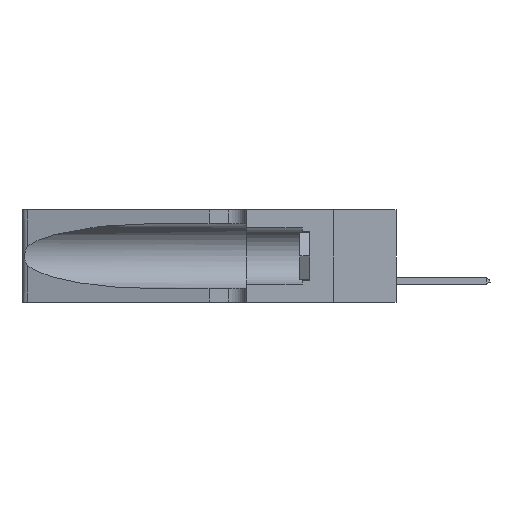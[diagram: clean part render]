
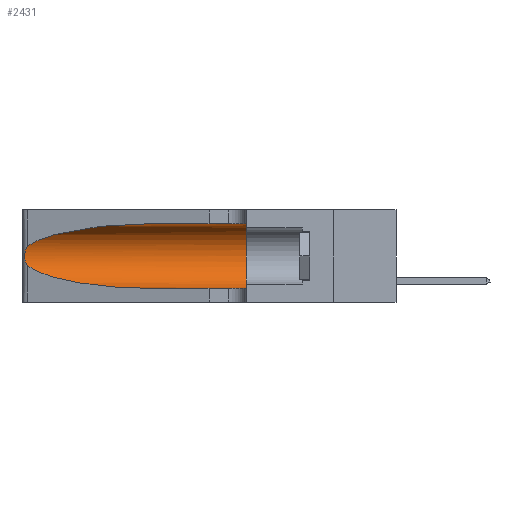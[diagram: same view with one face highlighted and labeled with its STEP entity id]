
A CAD part, left-side view. The second image highlights one B-rep face of the part: STEP entity #2431.
In plain terms, the highlighted cylindrical face has radius 3.308 mm (diameter 6.617 mm), a partial arc.
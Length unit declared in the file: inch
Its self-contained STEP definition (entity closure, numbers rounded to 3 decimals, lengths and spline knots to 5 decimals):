
#543 = CARTESIAN_POINT ( 'NONE',  ( 0.25856, 1.23593, 0.16098 ) ) ;
#841 = CARTESIAN_POINT ( 'NONE',  ( 0.25555, 1.22994, 0.2215 ) ) ;
#2431 = ADVANCED_FACE ( 'NONE', ( #20573 ), #27741, .F. ) ;
#2464 = EDGE_CURVE ( 'NONE', #37446, #22092, #39561, .T. ) ;
#2761 = EDGE_CURVE ( 'NONE', #19923, #37446, #9212, .T. ) ;
#3062 = CARTESIAN_POINT ( 'NONE',  ( 0.1305, 0.35, 0.185 ) ) ;
#3787 = CARTESIAN_POINT ( 'NONE',  ( 0.25639, 1.23184, 0.21858 ) ) ;
#3931 = CARTESIAN_POINT ( 'NONE',  ( 0.25639, 1.23186, 0.15144 ) ) ;
#4174 = VERTEX_POINT ( 'NONE', #24287 ) ;
#5239 = EDGE_CURVE ( 'NONE', #22092, #4174, #22584, .T. ) ;
#5716 = VECTOR ( 'NONE', #24794, 39.37008 ) ;
#5760 = VECTOR ( 'NONE', #39925, 39.37008 ) ;
#7243 = CARTESIAN_POINT ( 'NONE',  ( 0.26075, 1.23896, 0.178 ) ) ;
#7381 = CARTESIAN_POINT ( 'NONE',  ( 0.26017, 1.23833, 0.17102 ) ) ;
#7529 = CARTESIAN_POINT ( 'NONE',  ( 0.25487, 1.22718, 0.14631 ) ) ;
#9212 =( BOUNDED_CURVE ( )  B_SPLINE_CURVE ( 3, ( #34380, #21546, #33027, #35935 ),
 .UNSPECIFIED., .F., .F. ) 
 B_SPLINE_CURVE_WITH_KNOTS ( ( 4, 4 ),
 ( 1.5708, 2.84003 ),
 .UNSPECIFIED. ) 
 CURVE ( )  GEOMETRIC_REPRESENTATION_ITEM ( )  RATIONAL_B_SPLINE_CURVE ( ( 1., 0.87, 0.87, 1. ) ) 
 REPRESENTATION_ITEM ( '' )  );
#10047 = ORIENTED_EDGE ( 'NONE', *, *, #25328, .T. ) ;
#10255 = DIRECTION ( 'NONE',  ( 0., 0., -1. ) ) ;
#10950 = CARTESIAN_POINT ( 'NONE',  ( 0.26075, 1.23896, 0.19203 ) ) ;
#12093 = CARTESIAN_POINT ( 'NONE',  ( 0.25487, 1.22718, 0.14631 ) ) ;
#12885 = CARTESIAN_POINT ( 'NONE',  ( 0.18966, 0.96281, 0.05475 ) ) ;
#13194 = DIRECTION ( 'NONE',  ( 0., 1., 0. ) ) ;
#13235 = CARTESIAN_POINT ( 'NONE',  ( 0.1305, 0.72297, 0.05475 ) ) ;
#13467 = ORIENTED_EDGE ( 'NONE', *, *, #19697, .F. ) ;
#14350 = CARTESIAN_POINT ( 'NONE',  ( 0.1305, 1.61858, 0.31525 ) ) ;
#16114 = ORIENTED_EDGE ( 'NONE', *, *, #2761, .T. ) ;
#17792 = CARTESIAN_POINT ( 'NONE',  ( 0.1305, 0.35, 0.31525 ) ) ;
#19623 = CIRCLE ( 'NONE', #22662, 0.13025 ) ;
#19697 = EDGE_CURVE ( 'NONE', #19923, #32440, #25213, .T. ) ;
#19923 = VERTEX_POINT ( 'NONE', #24162 ) ;
#20248 = CARTESIAN_POINT ( 'NONE',  ( 0.25787, 1.23484, 0.2124 ) ) ;
#20573 = FACE_OUTER_BOUND ( 'NONE', #28814, .T. ) ;
#21546 = CARTESIAN_POINT ( 'NONE',  ( 0.18966, 0.96281, 0.31525 ) ) ;
#21591 = ORIENTED_EDGE ( 'NONE', *, *, #2464, .T. ) ;
#22092 = VERTEX_POINT ( 'NONE', #38915 ) ;
#22584 =( BOUNDED_CURVE ( )  B_SPLINE_CURVE ( 3, ( #12093, #30904, #12885, #13235 ),
 .UNSPECIFIED., .F., .F. ) 
 B_SPLINE_CURVE_WITH_KNOTS ( ( 4, 4 ),
 ( 3.44316, 4.71239 ),
 .UNSPECIFIED. ) 
 CURVE ( )  GEOMETRIC_REPRESENTATION_ITEM ( )  RATIONAL_B_SPLINE_CURVE ( ( 1., 0.87, 0.87, 1. ) ) 
 REPRESENTATION_ITEM ( '' )  );
#22662 = AXIS2_PLACEMENT_3D ( 'NONE', #3062, #13194, #42107 ) ;
#23553 = CARTESIAN_POINT ( 'NONE',  ( 0.25789, 1.23486, 0.15765 ) ) ;
#23884 = EDGE_CURVE ( 'NONE', #32440, #31363, #19623, .T. ) ;
#24162 = CARTESIAN_POINT ( 'NONE',  ( 0.1305, 0.72297, 0.31525 ) ) ;
#24287 = CARTESIAN_POINT ( 'NONE',  ( 0.1305, 0.72297, 0.05475 ) ) ;
#24794 = DIRECTION ( 'NONE',  ( 0., -1., 0. ) ) ;
#25213 = LINE ( 'NONE', #14350, #5760 ) ;
#25328 = EDGE_CURVE ( 'NONE', #4174, #31363, #30226, .T. ) ;
#25661 = CARTESIAN_POINT ( 'NONE',  ( 0.1305, 1.61858, 0.185 ) ) ;
#26197 = DIRECTION ( 'NONE',  ( 0., -1., 0. ) ) ;
#26833 = CARTESIAN_POINT ( 'NONE',  ( 0.25487, 1.22718, 0.22369 ) ) ;
#27741 = CYLINDRICAL_SURFACE ( 'NONE', #38291, 0.13025 ) ;
#28814 = EDGE_LOOP ( 'NONE', ( #16114, #21591, #30632, #10047, #33966, #13467 ) ) ;
#30108 = CARTESIAN_POINT ( 'NONE',  ( 0.25555, 1.22993, 0.14849 ) ) ;
#30226 = LINE ( 'NONE', #33341, #5716 ) ;
#30632 = ORIENTED_EDGE ( 'NONE', *, *, #5239, .T. ) ;
#30904 = CARTESIAN_POINT ( 'NONE',  ( 0.2373, 1.15595, 0.08982 ) ) ;
#31363 = VERTEX_POINT ( 'NONE', #35324 ) ;
#32440 = VERTEX_POINT ( 'NONE', #17792 ) ;
#33027 = CARTESIAN_POINT ( 'NONE',  ( 0.2373, 1.15595, 0.28018 ) ) ;
#33341 = CARTESIAN_POINT ( 'NONE',  ( 0.1305, 1.61858, 0.05475 ) ) ;
#33832 = CARTESIAN_POINT ( 'NONE',  ( 0.26018, 1.23835, 0.19895 ) ) ;
#33966 = ORIENTED_EDGE ( 'NONE', *, *, #23884, .F. ) ;
#34380 = CARTESIAN_POINT ( 'NONE',  ( 0.1305, 0.72297, 0.31525 ) ) ;
#35324 = CARTESIAN_POINT ( 'NONE',  ( 0.1305, 0.35, 0.05475 ) ) ;
#35935 = CARTESIAN_POINT ( 'NONE',  ( 0.25487, 1.22718, 0.22369 ) ) ;
#36958 = CARTESIAN_POINT ( 'NONE',  ( 0.25854, 1.2359, 0.20912 ) ) ;
#37446 = VERTEX_POINT ( 'NONE', #41481 ) ;
#38291 = AXIS2_PLACEMENT_3D ( 'NONE', #25661, #26197, #10255 ) ;
#38915 = CARTESIAN_POINT ( 'NONE',  ( 0.25487, 1.22718, 0.14631 ) ) ;
#39561 = B_SPLINE_CURVE_WITH_KNOTS ( 'NONE', 3,
 ( #26833, #841, #3787, #20248, #36958, #33832, #10950, #7243, #7381, #543, #23553, #3931, #30108, #7529 ),
 .UNSPECIFIED., .F., .F.,
 ( 4, 2, 2, 2, 2, 2, 4 ),
 ( 0., 0.00027, 0.00053, 0.00107, 0.0016, 0.00187, 0.00214 ),
 .UNSPECIFIED. ) ;
#39925 = DIRECTION ( 'NONE',  ( 0., -1., 0. ) ) ;
#41481 = CARTESIAN_POINT ( 'NONE',  ( 0.25487, 1.22718, 0.22369 ) ) ;
#42107 = DIRECTION ( 'NONE',  ( 0., 0., 1. ) ) ;
